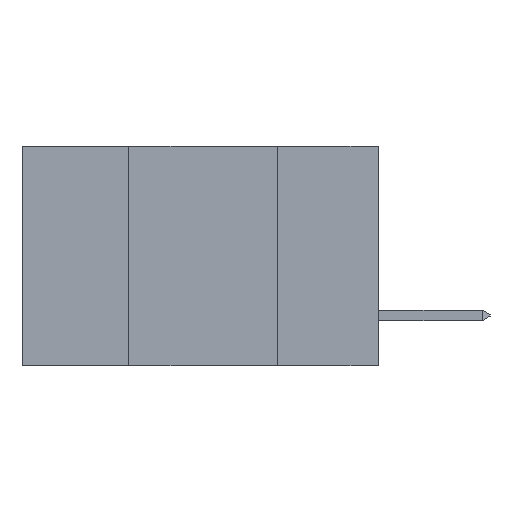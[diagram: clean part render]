
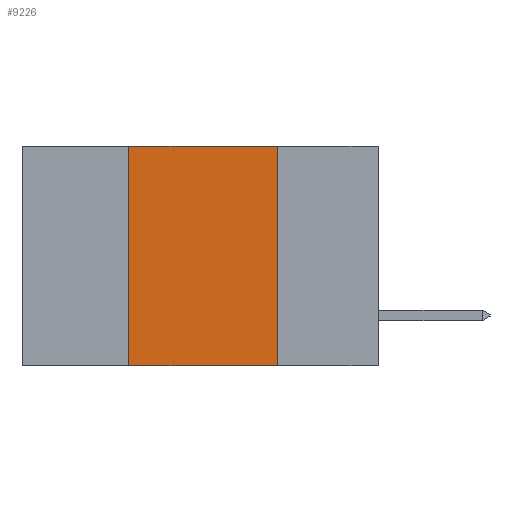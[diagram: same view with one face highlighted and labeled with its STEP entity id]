
A CAD part, left-side view. The second image highlights one B-rep face of the part: STEP entity #9226.
In plain terms, the highlighted planar face has unit normal (-1, 0, 0).
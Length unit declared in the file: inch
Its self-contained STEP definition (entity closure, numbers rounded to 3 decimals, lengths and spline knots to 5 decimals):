
#175 = ORIENTED_EDGE ( 'NONE', *, *, #16558, .F. ) ;
#910 = CARTESIAN_POINT ( 'NONE',  ( 0., 0.17, 0. ) ) ;
#1099 = CARTESIAN_POINT ( 'NONE',  ( 0., 0.17, -0.37 ) ) ;
#1384 = CARTESIAN_POINT ( 'NONE',  ( 0., 0.42, -0.37 ) ) ;
#2087 = DIRECTION ( 'NONE',  ( 0., -1., 0. ) ) ;
#2107 = CARTESIAN_POINT ( 'NONE',  ( 0., 0.17, -0.37 ) ) ;
#3622 = CARTESIAN_POINT ( 'NONE',  ( 0., 0.6, 0. ) ) ;
#4109 = VECTOR ( 'NONE', #14828, 39.37008 ) ;
#4322 = CARTESIAN_POINT ( 'NONE',  ( 0., 0.42, -0.37 ) ) ;
#5969 = VECTOR ( 'NONE', #2087, 39.37008 ) ;
#6489 = AXIS2_PLACEMENT_3D ( 'NONE', #15875, #15832, #15762 ) ;
#6913 = LINE ( 'NONE', #3622, #5969 ) ;
#7301 = ORIENTED_EDGE ( 'NONE', *, *, #10840, .T. ) ;
#7543 = CARTESIAN_POINT ( 'NONE',  ( 0., 0.42, 0. ) ) ;
#8147 = VECTOR ( 'NONE', #8944, 39.37008 ) ;
#8431 = VERTEX_POINT ( 'NONE', #910 ) ;
#8907 = VERTEX_POINT ( 'NONE', #7543 ) ;
#8944 = DIRECTION ( 'NONE',  ( 0., 0., 1. ) ) ;
#9038 = EDGE_LOOP ( 'NONE', ( #19833, #9815, #175, #7301 ) ) ;
#9226 = ADVANCED_FACE ( 'NONE', ( #16983 ), #16126, .F. ) ;
#9815 = ORIENTED_EDGE ( 'NONE', *, *, #11391, .F. ) ;
#10840 = EDGE_CURVE ( 'NONE', #11073, #10947, #19997, .T. ) ;
#10947 = VERTEX_POINT ( 'NONE', #1099 ) ;
#11073 = VERTEX_POINT ( 'NONE', #1384 ) ;
#11343 = DIRECTION ( 'NONE',  ( 0., 0., -1. ) ) ;
#11391 = EDGE_CURVE ( 'NONE', #8907, #8431, #6913, .T. ) ;
#14247 = VECTOR ( 'NONE', #11343, 39.37008 ) ;
#14768 = LINE ( 'NONE', #2107, #14247 ) ;
#14828 = DIRECTION ( 'NONE',  ( 0., -1., 0. ) ) ;
#14890 = EDGE_CURVE ( 'NONE', #8431, #10947, #14768, .T. ) ;
#15762 = DIRECTION ( 'NONE',  ( 0., 0., -1. ) ) ;
#15832 = DIRECTION ( 'NONE',  ( 1., 0., 0. ) ) ;
#15875 = CARTESIAN_POINT ( 'NONE',  ( 0., 0.6, 0. ) ) ;
#15932 = LINE ( 'NONE', #4322, #8147 ) ;
#16126 = PLANE ( 'NONE',  #6489 ) ;
#16558 = EDGE_CURVE ( 'NONE', #11073, #8907, #15932, .T. ) ;
#16983 = FACE_OUTER_BOUND ( 'NONE', #9038, .T. ) ;
#17901 = CARTESIAN_POINT ( 'NONE',  ( 0., 0.6, -0.37 ) ) ;
#19833 = ORIENTED_EDGE ( 'NONE', *, *, #14890, .F. ) ;
#19997 = LINE ( 'NONE', #17901, #4109 ) ;
